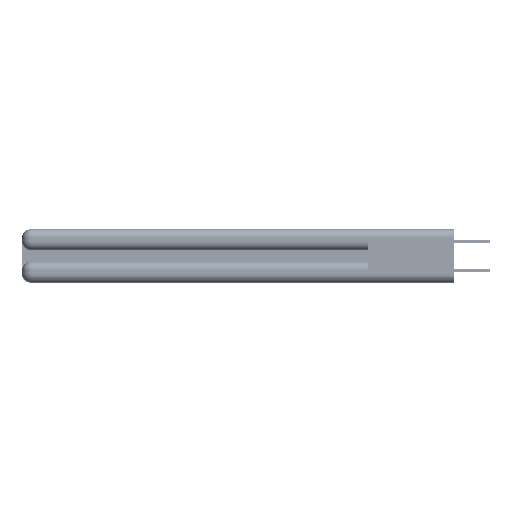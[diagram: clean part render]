
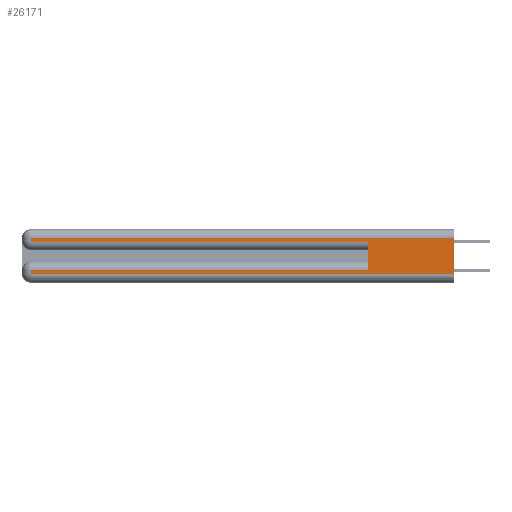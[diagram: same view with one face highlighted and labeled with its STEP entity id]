
A CAD part, left-side view. The second image highlights one B-rep face of the part: STEP entity #26171.
In plain terms, the highlighted planar face has unit normal (-1, 0, 0).
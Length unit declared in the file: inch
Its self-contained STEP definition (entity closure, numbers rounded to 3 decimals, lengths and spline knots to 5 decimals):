
#800 = DIRECTION ( 'NONE',  ( 0., -1., 0. ) ) ;
#1811 = EDGE_CURVE ( 'NONE', #26205, #20223, #35943, .T. ) ;
#5784 = VERTEX_POINT ( 'NONE', #17529 ) ;
#6426 = LINE ( 'NONE', #13703, #50811 ) ;
#7060 = VECTOR ( 'NONE', #47927, 39.37008 ) ;
#9601 = LINE ( 'NONE', #26509, #27791 ) ;
#11126 = LINE ( 'NONE', #28540, #54789 ) ;
#12060 = ORIENTED_EDGE ( 'NONE', *, *, #49852, .F. ) ;
#13703 = CARTESIAN_POINT ( 'NONE',  ( 0., 2.94, 0.37 ) ) ;
#14579 = EDGE_CURVE ( 'NONE', #20223, #38902, #11126, .T. ) ;
#14582 = ORIENTED_EDGE ( 'NONE', *, *, #14579, .T. ) ;
#15701 = VERTEX_POINT ( 'NONE', #25969 ) ;
#16455 = LINE ( 'NONE', #50277, #30590 ) ;
#16497 = LINE ( 'NONE', #17524, #7060 ) ;
#17524 = CARTESIAN_POINT ( 'NONE',  ( 0., 0., 0.06 ) ) ;
#17529 = CARTESIAN_POINT ( 'NONE',  ( 0., 0.6, 0.285 ) ) ;
#18650 = CARTESIAN_POINT ( 'NONE',  ( 0., 2.94, 0.085 ) ) ;
#19420 = VERTEX_POINT ( 'NONE', #18650 ) ;
#19805 = VECTOR ( 'NONE', #53873, 39.37008 ) ;
#20040 = CARTESIAN_POINT ( 'NONE',  ( 0., 2.94, 0.31 ) ) ;
#20223 = VERTEX_POINT ( 'NONE', #20040 ) ;
#22319 = DIRECTION ( 'NONE',  ( 0., 0., -1. ) ) ;
#23763 = ORIENTED_EDGE ( 'NONE', *, *, #38074, .T. ) ;
#23828 = LINE ( 'NONE', #45959, #19805 ) ;
#24011 = DIRECTION ( 'NONE',  ( 0., 1., 0. ) ) ;
#24166 = DIRECTION ( 'NONE',  ( 0., 1., 0. ) ) ;
#24242 = ORIENTED_EDGE ( 'NONE', *, *, #1811, .T. ) ;
#24474 = VECTOR ( 'NONE', #24011, 39.37008 ) ;
#24667 = CARTESIAN_POINT ( 'NONE',  ( 0., 2.94, 0.285 ) ) ;
#25533 = EDGE_CURVE ( 'NONE', #15701, #34381, #16497, .T. ) ;
#25603 = ORIENTED_EDGE ( 'NONE', *, *, #32496, .F. ) ;
#25969 = CARTESIAN_POINT ( 'NONE',  ( 0., 2.94, 0.06 ) ) ;
#26171 = ADVANCED_FACE ( 'NONE', ( #43265 ), #39044, .F. ) ;
#26205 = VERTEX_POINT ( 'NONE', #35123 ) ;
#26404 = EDGE_CURVE ( 'NONE', #44909, #19420, #16455, .T. ) ;
#26509 = CARTESIAN_POINT ( 'NONE',  ( 0., 0., 0.285 ) ) ;
#27457 = EDGE_CURVE ( 'NONE', #38902, #5784, #9601, .T. ) ;
#27791 = VECTOR ( 'NONE', #800, 39.37008 ) ;
#28540 = CARTESIAN_POINT ( 'NONE',  ( 0., 2.94, 0.37 ) ) ;
#30590 = VECTOR ( 'NONE', #24166, 39.37008 ) ;
#31360 = VECTOR ( 'NONE', #49532, 39.37008 ) ;
#32265 = CARTESIAN_POINT ( 'NONE',  ( 0., 0.6, 0.145 ) ) ;
#32496 = EDGE_CURVE ( 'NONE', #26205, #34381, #23828, .T. ) ;
#34381 = VERTEX_POINT ( 'NONE', #50472 ) ;
#34605 = AXIS2_PLACEMENT_3D ( 'NONE', #47707, #52000, #22319 ) ;
#35123 = CARTESIAN_POINT ( 'NONE',  ( 0., 0., 0.31 ) ) ;
#35943 = LINE ( 'NONE', #41107, #24474 ) ;
#38074 = EDGE_CURVE ( 'NONE', #19420, #15701, #6426, .T. ) ;
#38902 = VERTEX_POINT ( 'NONE', #24667 ) ;
#39044 = PLANE ( 'NONE',  #34605 ) ;
#40893 = ORIENTED_EDGE ( 'NONE', *, *, #26404, .T. ) ;
#41107 = CARTESIAN_POINT ( 'NONE',  ( 0., 0., 0.31 ) ) ;
#43265 = FACE_OUTER_BOUND ( 'NONE', #52873, .T. ) ;
#44449 = ORIENTED_EDGE ( 'NONE', *, *, #25533, .T. ) ;
#44909 = VERTEX_POINT ( 'NONE', #53001 ) ;
#45403 = DIRECTION ( 'NONE',  ( 0., 0., -1. ) ) ;
#45443 = LINE ( 'NONE', #32265, #31360 ) ;
#45959 = CARTESIAN_POINT ( 'NONE',  ( 0., 0., 0.37 ) ) ;
#47707 = CARTESIAN_POINT ( 'NONE',  ( 0., 0., 0.37 ) ) ;
#47927 = DIRECTION ( 'NONE',  ( 0., -1., 0. ) ) ;
#49532 = DIRECTION ( 'NONE',  ( 0., 0., 1. ) ) ;
#49852 = EDGE_CURVE ( 'NONE', #44909, #5784, #45443, .T. ) ;
#50277 = CARTESIAN_POINT ( 'NONE',  ( 0., 0., 0.085 ) ) ;
#50472 = CARTESIAN_POINT ( 'NONE',  ( 0., 0., 0.06 ) ) ;
#50811 = VECTOR ( 'NONE', #52743, 39.37008 ) ;
#52000 = DIRECTION ( 'NONE',  ( 1., 0., 0. ) ) ;
#52197 = ORIENTED_EDGE ( 'NONE', *, *, #27457, .T. ) ;
#52743 = DIRECTION ( 'NONE',  ( 0., 0., -1. ) ) ;
#52873 = EDGE_LOOP ( 'NONE', ( #25603, #24242, #14582, #52197, #12060, #40893, #23763, #44449 ) ) ;
#53001 = CARTESIAN_POINT ( 'NONE',  ( 0., 0.6, 0.085 ) ) ;
#53873 = DIRECTION ( 'NONE',  ( 0., 0., -1. ) ) ;
#54789 = VECTOR ( 'NONE', #45403, 39.37008 ) ;
